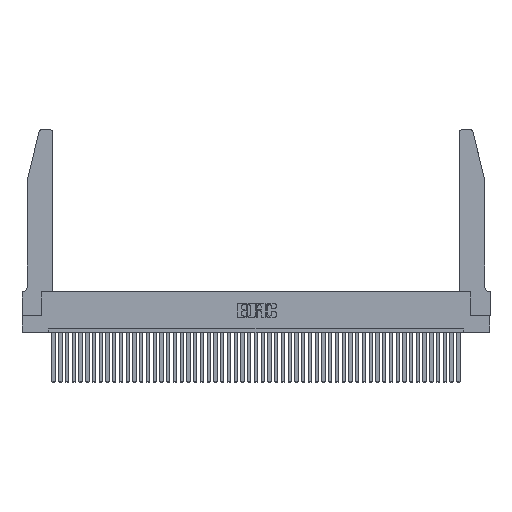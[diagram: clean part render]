
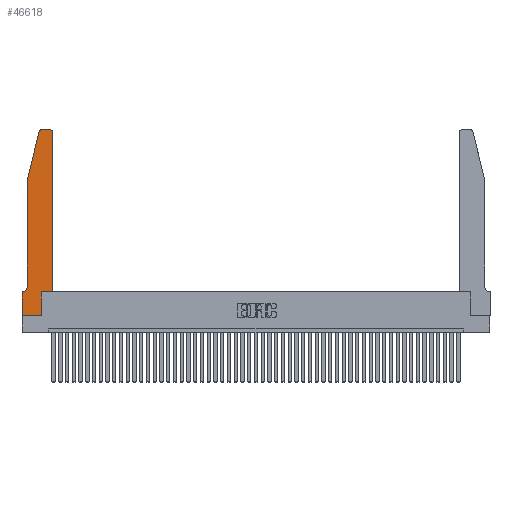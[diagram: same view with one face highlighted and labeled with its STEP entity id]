
A CAD part, top view. The second image highlights one B-rep face of the part: STEP entity #46618.
In plain terms, the highlighted planar face has unit normal (0, 0, 1).
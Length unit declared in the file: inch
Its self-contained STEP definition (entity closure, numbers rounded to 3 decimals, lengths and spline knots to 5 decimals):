
#50 = CARTESIAN_POINT ( 'NONE',  ( 0.2865, 0., 0.37 ) ) ;
#365 = VERTEX_POINT ( 'NONE', #21078 ) ;
#427 = VERTEX_POINT ( 'NONE', #50 ) ;
#654 = DIRECTION ( 'NONE',  ( 1., 0., 0. ) ) ;
#1286 = CARTESIAN_POINT ( 'NONE',  ( 0.4505, 0.35, 0.37 ) ) ;
#1738 = DIRECTION ( 'NONE',  ( 0., 0., 1. ) ) ;
#1831 = ORIENTED_EDGE ( 'NONE', *, *, #33635, .T. ) ;
#1979 = CIRCLE ( 'NONE', #17116, 0.03 ) ;
#2903 = DIRECTION ( 'NONE',  ( -0.239, -0.971, 0. ) ) ;
#2911 = DIRECTION ( 'NONE',  ( 0., -1., 0. ) ) ;
#2927 = CARTESIAN_POINT ( 'NONE',  ( 0.4505, 0.35, 0.37 ) ) ;
#3503 = DIRECTION ( 'NONE',  ( -1., 0., 0. ) ) ;
#3714 = VECTOR ( 'NONE', #4415, 39.37008 ) ;
#4415 = DIRECTION ( 'NONE',  ( 0., 1., 0. ) ) ;
#5121 = VECTOR ( 'NONE', #25610, 39.37008 ) ;
#5573 = ORIENTED_EDGE ( 'NONE', *, *, #24070, .T. ) ;
#5722 = LINE ( 'NONE', #16809, #38158 ) ;
#7607 = VERTEX_POINT ( 'NONE', #36589 ) ;
#7698 = VERTEX_POINT ( 'NONE', #10950 ) ;
#7747 = VERTEX_POINT ( 'NONE', #11326 ) ;
#8174 = VECTOR ( 'NONE', #2911, 39.37008 ) ;
#8884 = CARTESIAN_POINT ( 'NONE',  ( 0.0755, 0.42, 0.37 ) ) ;
#10116 = EDGE_LOOP ( 'NONE', ( #46379, #34163, #40952, #21423, #43303, #36529, #1831, #5573, #31342, #29044, #36293, #11053 ) ) ;
#10265 = CARTESIAN_POINT ( 'NONE',  ( 0.0755, 2., 0.37 ) ) ;
#10318 = CARTESIAN_POINT ( 'NONE',  ( 0.4505, 0.35, 0.37 ) ) ;
#10950 = CARTESIAN_POINT ( 'NONE',  ( 0.4505, 2.72, 0.37 ) ) ;
#11008 = CIRCLE ( 'NONE', #23312, 0.07 ) ;
#11053 = ORIENTED_EDGE ( 'NONE', *, *, #40427, .T. ) ;
#11326 = CARTESIAN_POINT ( 'NONE',  ( 0., 0.35, 0.37 ) ) ;
#11380 = CARTESIAN_POINT ( 'NONE',  ( 0.284, 2.72, 0.37 ) ) ;
#11794 = VERTEX_POINT ( 'NONE', #36401 ) ;
#11816 = DIRECTION ( 'NONE',  ( 0., 0., 1. ) ) ;
#12584 = DIRECTION ( 'NONE',  ( 1., 0., 0. ) ) ;
#12919 = DIRECTION ( 'NONE',  ( 0., 0., -1. ) ) ;
#14073 = CARTESIAN_POINT ( 'NONE',  ( 0.0755, 0.35, 0.37 ) ) ;
#14685 = DIRECTION ( 'NONE',  ( 0., 1., 0. ) ) ;
#15359 = FACE_OUTER_BOUND ( 'NONE', #10116, .T. ) ;
#15931 = CARTESIAN_POINT ( 'NONE',  ( 0.25487, 2.72718, 0.37 ) ) ;
#16077 = LINE ( 'NONE', #10265, #5121 ) ;
#16283 = PLANE ( 'NONE',  #28181 ) ;
#16317 = CARTESIAN_POINT ( 'NONE',  ( 0.2865, 0.35, 0.37 ) ) ;
#16412 = VERTEX_POINT ( 'NONE', #10318 ) ;
#16457 = CARTESIAN_POINT ( 'NONE',  ( 0.0055, 0.42, 0.37 ) ) ;
#16625 = DIRECTION ( 'NONE',  ( -1., 0., 0. ) ) ;
#16809 = CARTESIAN_POINT ( 'NONE',  ( 0., 0., 0.37 ) ) ;
#17116 = AXIS2_PLACEMENT_3D ( 'NONE', #11380, #44851, #33886 ) ;
#17621 = DIRECTION ( 'NONE',  ( -1., 0., 0. ) ) ;
#17916 = VERTEX_POINT ( 'NONE', #16317 ) ;
#18708 = EDGE_CURVE ( 'NONE', #46748, #47437, #11008, .T. ) ;
#19521 = EDGE_CURVE ( 'NONE', #7607, #46748, #16077, .T. ) ;
#21078 = CARTESIAN_POINT ( 'NONE',  ( 0., 0., 0.37 ) ) ;
#21423 = ORIENTED_EDGE ( 'NONE', *, *, #19521, .T. ) ;
#22157 = LINE ( 'NONE', #37492, #3714 ) ;
#22360 = LINE ( 'NONE', #14073, #22952 ) ;
#22815 = LINE ( 'NONE', #2927, #26892 ) ;
#22952 = VECTOR ( 'NONE', #17621, 39.37008 ) ;
#23312 = AXIS2_PLACEMENT_3D ( 'NONE', #16457, #12919, #16625 ) ;
#23902 = EDGE_CURVE ( 'NONE', #11794, #37242, #34661, .T. ) ;
#23907 = CARTESIAN_POINT ( 'NONE',  ( 0., 0.35, 0.37 ) ) ;
#24070 = EDGE_CURVE ( 'NONE', #365, #427, #5722, .T. ) ;
#24344 = CARTESIAN_POINT ( 'NONE',  ( 0.0055, 0.35, 0.37 ) ) ;
#25610 = DIRECTION ( 'NONE',  ( 0., -1., 0. ) ) ;
#26663 = LINE ( 'NONE', #39642, #8174 ) ;
#26770 = VERTEX_POINT ( 'NONE', #15931 ) ;
#26892 = VECTOR ( 'NONE', #28688, 39.37008 ) ;
#28181 = AXIS2_PLACEMENT_3D ( 'NONE', #23907, #1738, #31707 ) ;
#28283 = EDGE_CURVE ( 'NONE', #26770, #7607, #44540, .T. ) ;
#28688 = DIRECTION ( 'NONE',  ( 1., 0., 0. ) ) ;
#29044 = ORIENTED_EDGE ( 'NONE', *, *, #31219, .T. ) ;
#29846 = EDGE_CURVE ( 'NONE', #47437, #7747, #22360, .T. ) ;
#31219 = EDGE_CURVE ( 'NONE', #17916, #16412, #22815, .T. ) ;
#31333 = EDGE_CURVE ( 'NONE', #16412, #7698, #47753, .T. ) ;
#31342 = ORIENTED_EDGE ( 'NONE', *, *, #39605, .T. ) ;
#31707 = DIRECTION ( 'NONE',  ( 1., 0., 0. ) ) ;
#31795 = VECTOR ( 'NONE', #3503, 39.37008 ) ;
#33635 = EDGE_CURVE ( 'NONE', #7747, #365, #26663, .T. ) ;
#33886 = DIRECTION ( 'NONE',  ( 1., 0., 0. ) ) ;
#34163 = ORIENTED_EDGE ( 'NONE', *, *, #39624, .T. ) ;
#34661 = LINE ( 'NONE', #47809, #31795 ) ;
#36293 = ORIENTED_EDGE ( 'NONE', *, *, #31333, .T. ) ;
#36401 = CARTESIAN_POINT ( 'NONE',  ( 0.4205, 2.75, 0.37 ) ) ;
#36529 = ORIENTED_EDGE ( 'NONE', *, *, #29846, .T. ) ;
#36589 = CARTESIAN_POINT ( 'NONE',  ( 0.0755, 2., 0.37 ) ) ;
#37242 = VERTEX_POINT ( 'NONE', #45186 ) ;
#37492 = CARTESIAN_POINT ( 'NONE',  ( 0.2865, 0.35, 0.37 ) ) ;
#37621 = AXIS2_PLACEMENT_3D ( 'NONE', #45328, #11816, #654 ) ;
#38158 = VECTOR ( 'NONE', #12584, 39.37008 ) ;
#39307 = CARTESIAN_POINT ( 'NONE',  ( 0.0755, 2., 0.37 ) ) ;
#39605 = EDGE_CURVE ( 'NONE', #427, #17916, #22157, .T. ) ;
#39624 = EDGE_CURVE ( 'NONE', #37242, #26770, #1979, .T. ) ;
#39642 = CARTESIAN_POINT ( 'NONE',  ( 0., 0., 0.37 ) ) ;
#40427 = EDGE_CURVE ( 'NONE', #7698, #11794, #42958, .T. ) ;
#40952 = ORIENTED_EDGE ( 'NONE', *, *, #28283, .T. ) ;
#41298 = VECTOR ( 'NONE', #2903, 39.37008 ) ;
#42958 = CIRCLE ( 'NONE', #37621, 0.03 ) ;
#43303 = ORIENTED_EDGE ( 'NONE', *, *, #18708, .T. ) ;
#44540 = LINE ( 'NONE', #39307, #41298 ) ;
#44851 = DIRECTION ( 'NONE',  ( 0., 0., 1. ) ) ;
#45186 = CARTESIAN_POINT ( 'NONE',  ( 0.284, 2.75, 0.37 ) ) ;
#45328 = CARTESIAN_POINT ( 'NONE',  ( 0.4205, 2.72, 0.37 ) ) ;
#46009 = VECTOR ( 'NONE', #14685, 39.37008 ) ;
#46379 = ORIENTED_EDGE ( 'NONE', *, *, #23902, .T. ) ;
#46618 = ADVANCED_FACE ( 'NONE', ( #15359 ), #16283, .T. ) ;
#46748 = VERTEX_POINT ( 'NONE', #8884 ) ;
#47437 = VERTEX_POINT ( 'NONE', #24344 ) ;
#47753 = LINE ( 'NONE', #1286, #46009 ) ;
#47809 = CARTESIAN_POINT ( 'NONE',  ( 0.2605, 2.75, 0.37 ) ) ;
